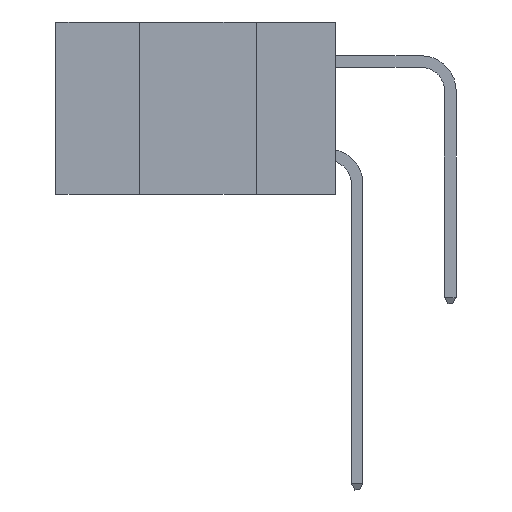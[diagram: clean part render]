
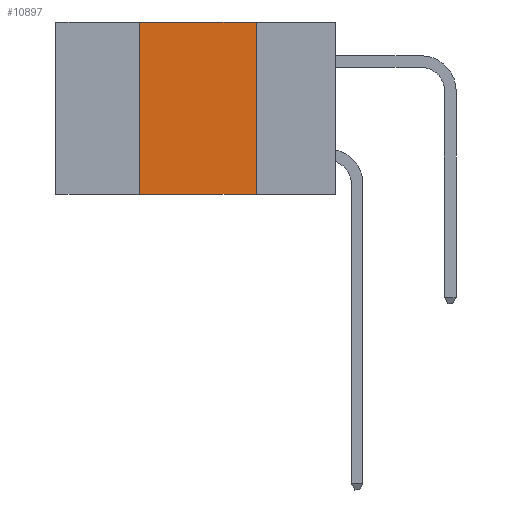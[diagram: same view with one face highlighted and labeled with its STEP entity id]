
A CAD part, left-side view. The second image highlights one B-rep face of the part: STEP entity #10897.
In plain terms, the highlighted planar face has unit normal (-1, 0, 0).
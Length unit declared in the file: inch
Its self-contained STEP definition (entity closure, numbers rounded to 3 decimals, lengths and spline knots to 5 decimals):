
#144 = DIRECTION ( 'NONE',  ( 1., 0., 0. ) ) ;
#882 = ORIENTED_EDGE ( 'NONE', *, *, #6571, .T. ) ;
#1306 = AXIS2_PLACEMENT_3D ( 'NONE', #3031, #144, #10045 ) ;
#3031 = CARTESIAN_POINT ( 'NONE',  ( 0., 0.6, 0. ) ) ;
#3968 = CARTESIAN_POINT ( 'NONE',  ( 0., 0.42, 0. ) ) ;
#4916 = ORIENTED_EDGE ( 'NONE', *, *, #11921, .F. ) ;
#5347 = VERTEX_POINT ( 'NONE', #17165 ) ;
#5423 = CARTESIAN_POINT ( 'NONE',  ( 0., 0.17, 0. ) ) ;
#5514 = VECTOR ( 'NONE', #9806, 39.37008 ) ;
#5819 = FACE_OUTER_BOUND ( 'NONE', #11884, .T. ) ;
#5820 = CARTESIAN_POINT ( 'NONE',  ( 0., 0.42, -0.37 ) ) ;
#6571 = EDGE_CURVE ( 'NONE', #7274, #17716, #9162, .T. ) ;
#7274 = VERTEX_POINT ( 'NONE', #5820 ) ;
#8407 = EDGE_CURVE ( 'NONE', #7274, #5347, #16375, .T. ) ;
#8654 = PLANE ( 'NONE',  #1306 ) ;
#8914 = VECTOR ( 'NONE', #12174, 39.37008 ) ;
#9162 = LINE ( 'NONE', #13729, #5514 ) ;
#9806 = DIRECTION ( 'NONE',  ( 0., -1., 0. ) ) ;
#9921 = ORIENTED_EDGE ( 'NONE', *, *, #8407, .F. ) ;
#10045 = DIRECTION ( 'NONE',  ( 0., 0., -1. ) ) ;
#10208 = LINE ( 'NONE', #11679, #16787 ) ;
#10333 = ORIENTED_EDGE ( 'NONE', *, *, #12847, .F. ) ;
#10897 = ADVANCED_FACE ( 'NONE', ( #5819 ), #8654, .F. ) ;
#11066 = VECTOR ( 'NONE', #13566, 39.37008 ) ;
#11190 = CARTESIAN_POINT ( 'NONE',  ( 0., 0.17, -0.37 ) ) ;
#11679 = CARTESIAN_POINT ( 'NONE',  ( 0., 0.6, 0. ) ) ;
#11884 = EDGE_LOOP ( 'NONE', ( #4916, #10333, #9921, #882 ) ) ;
#11921 = EDGE_CURVE ( 'NONE', #13251, #17716, #14966, .T. ) ;
#12174 = DIRECTION ( 'NONE',  ( 0., 0., 1. ) ) ;
#12847 = EDGE_CURVE ( 'NONE', #5347, #13251, #10208, .T. ) ;
#13251 = VERTEX_POINT ( 'NONE', #16378 ) ;
#13566 = DIRECTION ( 'NONE',  ( 0., 0., -1. ) ) ;
#13729 = CARTESIAN_POINT ( 'NONE',  ( 0., 0.6, -0.37 ) ) ;
#14966 = LINE ( 'NONE', #5423, #11066 ) ;
#16375 = LINE ( 'NONE', #3968, #8914 ) ;
#16378 = CARTESIAN_POINT ( 'NONE',  ( 0., 0.17, 0. ) ) ;
#16787 = VECTOR ( 'NONE', #16922, 39.37008 ) ;
#16922 = DIRECTION ( 'NONE',  ( 0., -1., 0. ) ) ;
#17165 = CARTESIAN_POINT ( 'NONE',  ( 0., 0.42, 0. ) ) ;
#17716 = VERTEX_POINT ( 'NONE', #11190 ) ;
